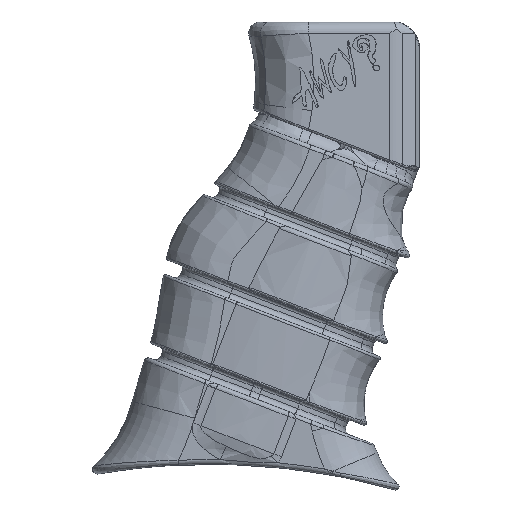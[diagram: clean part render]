
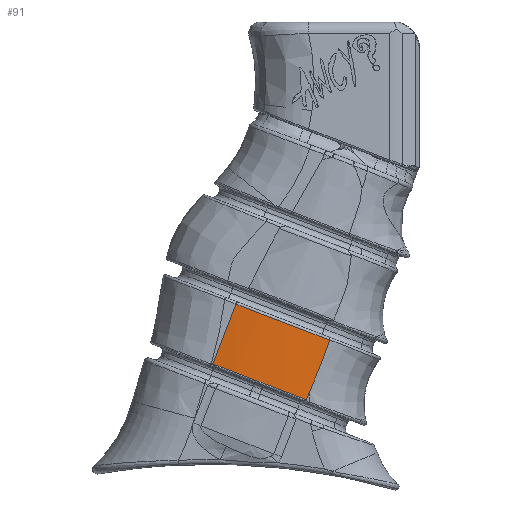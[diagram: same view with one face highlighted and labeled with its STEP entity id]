
A CAD part, front view. The second image highlights one B-rep face of the part: STEP entity #91.
In plain terms, the highlighted free-form (B-spline) face has degree [1, 2] with [2, 9] control points.
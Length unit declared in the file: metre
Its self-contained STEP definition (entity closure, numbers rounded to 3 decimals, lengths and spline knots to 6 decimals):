
#91=ADVANCED_FACE('0:111747',(#1010),#1011,.T.);
#1010=FACE_OUTER_BOUND('',#8261,.T.);
#1011=(B_SPLINE_SURFACE(1,2,((#8263,#8264,#8265,#8266,#8267,#8268,#8269,#8270,#8271),(#8272,#8273,#8274,#8275,#8276,#8277,#8278,#8279,#8280)),.UNSPECIFIED.,.F.,.T.,.F.)B_SPLINE_SURFACE_WITH_KNOTS((2,2),(3,2,2,2,3),(-0.890553,0.277089),(0.0,0.040582,0.081164,0.121746,0.162328),.UNSPECIFIED.)RATIONAL_B_SPLINE_SURFACE(((1.0,0.707,1.0,0.707,1.0,0.707,1.0,0.707,1.0),(1.0,0.707,1.0,0.707,1.0,0.707,1.0,0.707,1.0)))BOUNDED_SURFACE()REPRESENTATION_ITEM('')GEOMETRIC_REPRESENTATION_ITEM()SURFACE());
#8261=EDGE_LOOP('',(#70901,#70902,#70903,#70904,#70905));
#8263=CARTESIAN_POINT('',(-0.211001,-0.230332,0.113879));
#8264=CARTESIAN_POINT('',(-0.211001,-0.246952,0.113879));
#8265=CARTESIAN_POINT('',(-0.186882,-0.246952,0.10462));
#8266=CARTESIAN_POINT('',(-0.162763,-0.246952,0.095362));
#8267=CARTESIAN_POINT('',(-0.162763,-0.230332,0.095362));
#8268=CARTESIAN_POINT('',(-0.162763,-0.213713,0.095362));
#8269=CARTESIAN_POINT('',(-0.186882,-0.213713,0.10462));
#8270=CARTESIAN_POINT('',(-0.211001,-0.213713,0.113879));
#8271=CARTESIAN_POINT('',(-0.211001,-0.230332,0.113879));
#8272=CARTESIAN_POINT('',(-0.221812,-0.230332,0.085716));
#8273=CARTESIAN_POINT('',(-0.221812,-0.246952,0.085716));
#8274=CARTESIAN_POINT('',(-0.197693,-0.246952,0.076457));
#8275=CARTESIAN_POINT('',(-0.173574,-0.246952,0.067199));
#8276=CARTESIAN_POINT('',(-0.173573,-0.230332,0.067199));
#8277=CARTESIAN_POINT('',(-0.173573,-0.213713,0.067199));
#8278=CARTESIAN_POINT('',(-0.197693,-0.213713,0.076457));
#8279=CARTESIAN_POINT('',(-0.221812,-0.213713,0.085716));
#8280=CARTESIAN_POINT('',(-0.221812,-0.230332,0.085716));
#70901=ORIENTED_EDGE('',*,*,#78380,.F.);
#70902=ORIENTED_EDGE('',*,*,#78381,.F.);
#70903=ORIENTED_EDGE('',*,*,#78382,.F.);
#70904=ORIENTED_EDGE('',*,*,#78383,.F.);
#70905=ORIENTED_EDGE('',*,*,#78384,.F.);
#78380=EDGE_CURVE('7:59069',#80912,#80903,#80914,.T.);
#78381=EDGE_CURVE('0:115499',#80915,#80912,#80916,.T.);
#78382=EDGE_CURVE('0:115508',#80917,#80915,#80918,.T.);
#78383=EDGE_CURVE('0:115472',#80919,#80917,#80920,.T.);
#78384=EDGE_CURVE('0:115505',#80903,#80919,#80921,.T.);
#80903=VERTEX_POINT('',#85952);
#80912=VERTEX_POINT('',#86010);
#80914=B_SPLINE_CURVE_WITH_KNOTS('',3,(#86021,#86022,#86023,#86024,#86025,#86026,#86027,#86028,#86029,#86030,#86031,#86032,#86033,#86034,#86035,#86036,#86037,#86038,#86039,#86040),.UNSPECIFIED.,.F.,.F.,(4,2,2,2,2,2,2,2,2,4),(-0.023852,-0.019539,-0.016326,-0.014317,-0.01269,-0.011063,-0.00846,-0.004295,-0.002148,-0.001531),.UNSPECIFIED.);
#80915=VERTEX_POINT('',#86041);
#80916=LINE('',#86042,#86043);
#80917=VERTEX_POINT('',#86044);
#80918=B_SPLINE_CURVE_WITH_KNOTS('',3,(#86045,#86046,#86047,#86048,#86049,#86050,#86051,#86052,#86053,#86054,#86055,#86056,#86057,#86058,#86059,#86060,#86061,#86062,#86063,#86064,#86065,#86066,#86067,#86068,#86069,#86070,#86071,#86072,#86073,#86074,#86075),.UNSPECIFIED.,.F.,.F.,(4,3,3,3,3,3,3,3,3,3,4),(0.000566,0.001194,0.003943,0.005006,0.006009,0.006449,0.007556,0.007982,0.009549,0.012027,0.012121),.UNSPECIFIED.);
#80919=VERTEX_POINT('',#86076);
#80920=ELLIPSE('',#86077,0.025843,0.01663);
#80921=LINE('',#86078,#86079);
#85952=CARTESIAN_POINT('',(-0.205376,-0.245315,0.087642));
#86010=CARTESIAN_POINT('',(-0.184499,-0.245315,0.079628));
#86021=CARTESIAN_POINT('',(-0.184499,-0.245315,0.079628));
#86022=CARTESIAN_POINT('',(-0.185801,-0.245746,0.080128));
#86023=CARTESIAN_POINT('',(-0.187133,-0.246087,0.080639));
#86024=CARTESIAN_POINT('',(-0.189482,-0.246537,0.081541));
#86025=CARTESIAN_POINT('',(-0.190493,-0.246683,0.081929));
#86026=CARTESIAN_POINT('',(-0.19214,-0.246846,0.082561));
#86027=CARTESIAN_POINT('',(-0.192774,-0.246891,0.082805));
#86028=CARTESIAN_POINT('',(-0.193921,-0.246941,0.083245));
#86029=CARTESIAN_POINT('',(-0.194434,-0.246952,0.083442));
#86030=CARTESIAN_POINT('',(-0.195457,-0.246952,0.083835));
#86031=CARTESIAN_POINT('',(-0.19597,-0.246941,0.084032));
#86032=CARTESIAN_POINT('',(-0.197304,-0.246882,0.084544));
#86033=CARTESIAN_POINT('',(-0.198126,-0.246816,0.084859));
#86034=CARTESIAN_POINT('',(-0.200255,-0.246569,0.085677));
#86035=CARTESIAN_POINT('',(-0.201559,-0.246341,0.086177));
#86036=CARTESIAN_POINT('',(-0.203508,-0.245875,0.086925));
#86037=CARTESIAN_POINT('',(-0.204165,-0.245695,0.087178));
#86038=CARTESIAN_POINT('',(-0.205003,-0.245436,0.087499));
#86039=CARTESIAN_POINT('',(-0.20519,-0.245376,0.087571));
#86040=CARTESIAN_POINT('',(-0.205376,-0.245315,0.087642));
#86041=CARTESIAN_POINT('',(-0.183758,-0.245315,0.081558));
#86042=CARTESIAN_POINT('',(-0.183758,-0.245315,0.081558));
#86043=VECTOR('',#102917,1.0);
#86044=CARTESIAN_POINT('',(-0.179335,-0.245302,0.092961));
#86045=CARTESIAN_POINT('',(-0.179335,-0.245302,0.092961));
#86046=CARTESIAN_POINT('',(-0.179403,-0.2453,0.092768));
#86047=CARTESIAN_POINT('',(-0.179469,-0.245298,0.092576));
#86048=CARTESIAN_POINT('',(-0.179534,-0.245295,0.092385));
#86049=CARTESIAN_POINT('',(-0.179822,-0.245286,0.091549));
#86050=CARTESIAN_POINT('',(-0.180098,-0.245275,0.090731));
#86051=CARTESIAN_POINT('',(-0.180406,-0.245268,0.089867));
#86052=CARTESIAN_POINT('',(-0.180525,-0.245265,0.089533));
#86053=CARTESIAN_POINT('',(-0.180649,-0.245263,0.089193));
#86054=CARTESIAN_POINT('',(-0.180781,-0.245262,0.088841));
#86055=CARTESIAN_POINT('',(-0.180905,-0.245261,0.08851));
#86056=CARTESIAN_POINT('',(-0.181037,-0.245261,0.088165));
#86057=CARTESIAN_POINT('',(-0.181171,-0.245262,0.087826));
#86058=CARTESIAN_POINT('',(-0.181229,-0.245263,0.087677));
#86059=CARTESIAN_POINT('',(-0.181289,-0.245263,0.087527));
#86060=CARTESIAN_POINT('',(-0.181349,-0.245264,0.087379));
#86061=CARTESIAN_POINT('',(-0.181499,-0.245266,0.087005));
#86062=CARTESIAN_POINT('',(-0.181651,-0.245269,0.086634));
#86063=CARTESIAN_POINT('',(-0.181807,-0.245273,0.086262));
#86064=CARTESIAN_POINT('',(-0.181867,-0.245274,0.086118));
#86065=CARTESIAN_POINT('',(-0.181927,-0.245276,0.085976));
#86066=CARTESIAN_POINT('',(-0.181988,-0.245277,0.085833));
#86067=CARTESIAN_POINT('',(-0.182209,-0.245283,0.085309));
#86068=CARTESIAN_POINT('',(-0.182431,-0.24529,0.084791));
#86069=CARTESIAN_POINT('',(-0.182655,-0.245296,0.084264));
#86070=CARTESIAN_POINT('',(-0.183009,-0.245306,0.08343));
#86071=CARTESIAN_POINT('',(-0.183368,-0.245314,0.08257));
#86072=CARTESIAN_POINT('',(-0.183718,-0.245315,0.081662));
#86073=CARTESIAN_POINT('',(-0.183732,-0.245315,0.081627));
#86074=CARTESIAN_POINT('',(-0.183745,-0.245315,0.081593));
#86075=CARTESIAN_POINT('',(-0.183758,-0.245315,0.081558));
#86076=CARTESIAN_POINT('',(-0.200252,-0.245315,0.10099));
#86077=AXIS2_PLACEMENT_3D('',#102918,#102919,#102920);
#86078=CARTESIAN_POINT('',(-0.20553,-0.245315,0.087241));
#86079=VECTOR('',#102921,1.0);
#102917=DIRECTION('',(-0.358,0.,-0.934));
#102918=CARTESIAN_POINT('',(-0.189813,-0.230322,0.096983));
#102919=DIRECTION('',(0.358,0.,0.934));
#102920=DIRECTION('',(0.934,0.,-0.358));
#102921=DIRECTION('',(0.358,0.,0.934));
